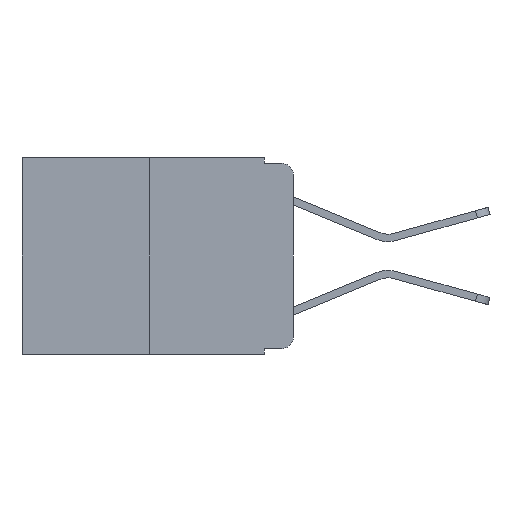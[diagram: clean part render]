
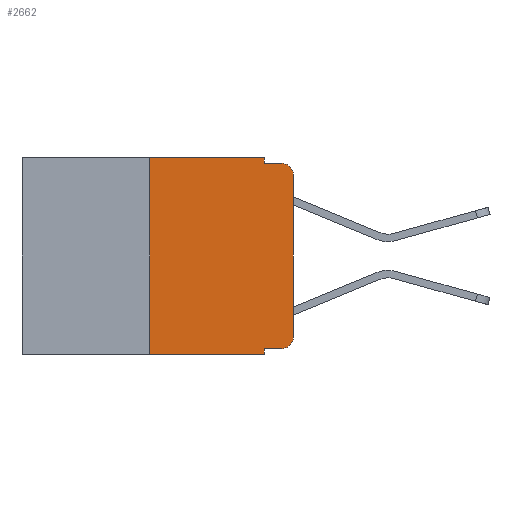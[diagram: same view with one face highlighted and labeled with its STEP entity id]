
A CAD part, left-side view. The second image highlights one B-rep face of the part: STEP entity #2662.
In plain terms, the highlighted planar face has unit normal (-1, 0, 0).
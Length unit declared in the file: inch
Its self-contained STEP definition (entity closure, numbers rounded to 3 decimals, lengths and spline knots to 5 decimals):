
#41 = EDGE_LOOP ( 'NONE', ( #711, #2804, #10533, #83, #5543, #851, #3449, #9483, #9194, #12041 ) ) ;
#83 = ORIENTED_EDGE ( 'NONE', *, *, #8245, .F. ) ;
#323 = VECTOR ( 'NONE', #6385, 39.37008 ) ;
#387 = EDGE_CURVE ( 'NONE', #10899, #10259, #6923, .T. ) ;
#709 = VECTOR ( 'NONE', #11092, 39.37008 ) ;
#711 = ORIENTED_EDGE ( 'NONE', *, *, #1309, .T. ) ;
#851 = ORIENTED_EDGE ( 'NONE', *, *, #9554, .F. ) ;
#940 = EDGE_CURVE ( 'NONE', #2561, #7400, #9088, .T. ) ;
#1270 = CARTESIAN_POINT ( 'NONE',  ( 0., 0.02, -0.01 ) ) ;
#1309 = EDGE_CURVE ( 'NONE', #5837, #7118, #4007, .T. ) ;
#1534 = AXIS2_PLACEMENT_3D ( 'NONE', #1995, #9180, #3088 ) ;
#1995 = CARTESIAN_POINT ( 'NONE',  ( 0., 0.02, -0.313 ) ) ;
#2171 = EDGE_CURVE ( 'NONE', #2561, #10259, #5730, .T. ) ;
#2261 = AXIS2_PLACEMENT_3D ( 'NONE', #2284, #9440, #3355 ) ;
#2284 = CARTESIAN_POINT ( 'NONE',  ( 0., 0.02, -0.03 ) ) ;
#2544 = DIRECTION ( 'NONE',  ( 1., 0., 0. ) ) ;
#2561 = VERTEX_POINT ( 'NONE', #8217 ) ;
#2662 = ADVANCED_FACE ( 'NONE', ( #4759 ), #9226, .F. ) ;
#2695 = CIRCLE ( 'NONE', #1534, 0.02 ) ;
#2804 = ORIENTED_EDGE ( 'NONE', *, *, #9386, .T. ) ;
#2941 = CARTESIAN_POINT ( 'NONE',  ( 0., 0.051, 0. ) ) ;
#3088 = DIRECTION ( 'NONE',  ( 0., 0., -1. ) ) ;
#3355 = DIRECTION ( 'NONE',  ( 0., 0., -1. ) ) ;
#3384 = CARTESIAN_POINT ( 'NONE',  ( 0., 0.473, 0. ) ) ;
#3437 = EDGE_CURVE ( 'NONE', #6474, #6135, #12771, .T. ) ;
#3449 = ORIENTED_EDGE ( 'NONE', *, *, #387, .T. ) ;
#3596 = LINE ( 'NONE', #6747, #8398 ) ;
#3625 = DIRECTION ( 'NONE',  ( 0., 0., 1. ) ) ;
#4007 = LINE ( 'NONE', #4478, #323 ) ;
#4095 = LINE ( 'NONE', #10329, #12298 ) ;
#4478 = CARTESIAN_POINT ( 'NONE',  ( 0., 0., 0. ) ) ;
#4759 = FACE_OUTER_BOUND ( 'NONE', #41, .T. ) ;
#4762 = EDGE_CURVE ( 'NONE', #13239, #12726, #4095, .T. ) ;
#5537 = VECTOR ( 'NONE', #5934, 39.37008 ) ;
#5543 = ORIENTED_EDGE ( 'NONE', *, *, #3437, .F. ) ;
#5546 = VECTOR ( 'NONE', #6477, 39.37008 ) ;
#5730 = LINE ( 'NONE', #8123, #11017 ) ;
#5837 = VERTEX_POINT ( 'NONE', #13210 ) ;
#5934 = DIRECTION ( 'NONE',  ( 0., -1., 0. ) ) ;
#5938 = CARTESIAN_POINT ( 'NONE',  ( 0., 0.473, 0. ) ) ;
#5997 = CARTESIAN_POINT ( 'NONE',  ( 0., 0.051, -0.343 ) ) ;
#6135 = VERTEX_POINT ( 'NONE', #2941 ) ;
#6362 = DIRECTION ( 'NONE',  ( 0., -1., 0. ) ) ;
#6385 = DIRECTION ( 'NONE',  ( 0., 0., 1. ) ) ;
#6474 = VERTEX_POINT ( 'NONE', #9891 ) ;
#6477 = DIRECTION ( 'NONE',  ( 0., 0., -1. ) ) ;
#6747 = CARTESIAN_POINT ( 'NONE',  ( 0., 0.25, 0. ) ) ;
#6923 = LINE ( 'NONE', #8673, #9267 ) ;
#7118 = VERTEX_POINT ( 'NONE', #7693 ) ;
#7257 = DIRECTION ( 'NONE',  ( 0., 0., -1. ) ) ;
#7400 = VERTEX_POINT ( 'NONE', #13046 ) ;
#7693 = CARTESIAN_POINT ( 'NONE',  ( 0., 0., -0.03 ) ) ;
#8123 = CARTESIAN_POINT ( 'NONE',  ( 0., 0.051, 0. ) ) ;
#8173 = AXIS2_PLACEMENT_3D ( 'NONE', #3384, #2544, #9451 ) ;
#8217 = CARTESIAN_POINT ( 'NONE',  ( 0., 0.051, -0.333 ) ) ;
#8245 = EDGE_CURVE ( 'NONE', #6135, #13239, #10855, .T. ) ;
#8246 = CIRCLE ( 'NONE', #2261, 0.02 ) ;
#8398 = VECTOR ( 'NONE', #3625, 39.37008 ) ;
#8673 = CARTESIAN_POINT ( 'NONE',  ( 0., 0.473, -0.343 ) ) ;
#9088 = LINE ( 'NONE', #11104, #709 ) ;
#9180 = DIRECTION ( 'NONE',  ( -1., 0., 0. ) ) ;
#9194 = ORIENTED_EDGE ( 'NONE', *, *, #940, .T. ) ;
#9226 = PLANE ( 'NONE',  #8173 ) ;
#9267 = VECTOR ( 'NONE', #13045, 39.37008 ) ;
#9386 = EDGE_CURVE ( 'NONE', #7118, #12726, #8246, .T. ) ;
#9440 = DIRECTION ( 'NONE',  ( -1., 0., 0. ) ) ;
#9451 = DIRECTION ( 'NONE',  ( 0., 0., -1. ) ) ;
#9483 = ORIENTED_EDGE ( 'NONE', *, *, #2171, .F. ) ;
#9554 = EDGE_CURVE ( 'NONE', #10899, #6474, #3596, .T. ) ;
#9891 = CARTESIAN_POINT ( 'NONE',  ( 0., 0.25, 0. ) ) ;
#9971 = CARTESIAN_POINT ( 'NONE',  ( 0., 0.25, -0.343 ) ) ;
#10259 = VERTEX_POINT ( 'NONE', #5997 ) ;
#10329 = CARTESIAN_POINT ( 'NONE',  ( 0., 0.051, -0.01 ) ) ;
#10533 = ORIENTED_EDGE ( 'NONE', *, *, #4762, .F. ) ;
#10855 = LINE ( 'NONE', #12316, #5546 ) ;
#10899 = VERTEX_POINT ( 'NONE', #9971 ) ;
#11017 = VECTOR ( 'NONE', #7257, 39.37008 ) ;
#11092 = DIRECTION ( 'NONE',  ( 0., -1., 0. ) ) ;
#11104 = CARTESIAN_POINT ( 'NONE',  ( 0., 0.051, -0.333 ) ) ;
#11310 = CARTESIAN_POINT ( 'NONE',  ( 0., 0.051, -0.01 ) ) ;
#12041 = ORIENTED_EDGE ( 'NONE', *, *, #13086, .T. ) ;
#12298 = VECTOR ( 'NONE', #6362, 39.37008 ) ;
#12316 = CARTESIAN_POINT ( 'NONE',  ( 0., 0.051, 0. ) ) ;
#12726 = VERTEX_POINT ( 'NONE', #1270 ) ;
#12771 = LINE ( 'NONE', #5938, #5537 ) ;
#13045 = DIRECTION ( 'NONE',  ( 0., -1., 0. ) ) ;
#13046 = CARTESIAN_POINT ( 'NONE',  ( 0., 0.02, -0.333 ) ) ;
#13086 = EDGE_CURVE ( 'NONE', #7400, #5837, #2695, .T. ) ;
#13210 = CARTESIAN_POINT ( 'NONE',  ( 0., 0., -0.313 ) ) ;
#13239 = VERTEX_POINT ( 'NONE', #11310 ) ;
